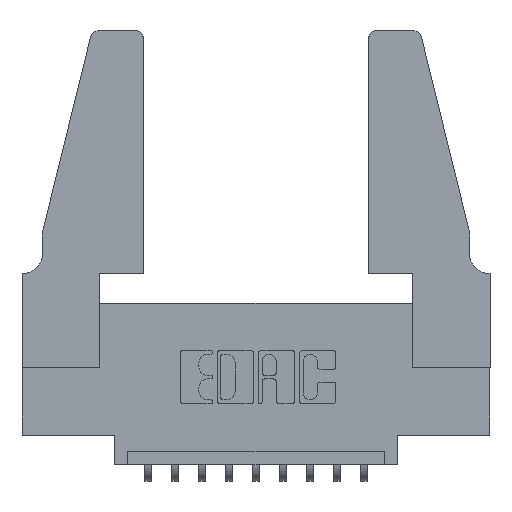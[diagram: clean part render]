
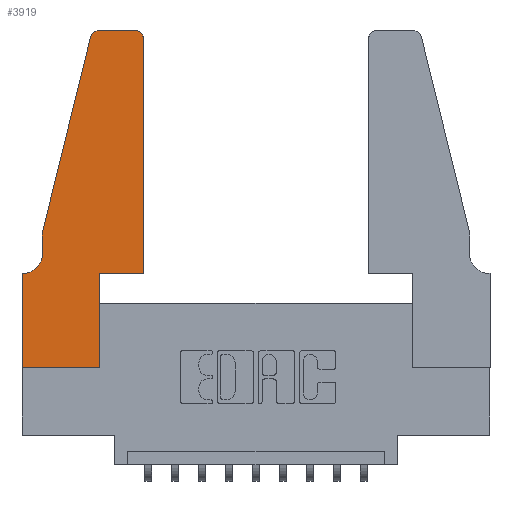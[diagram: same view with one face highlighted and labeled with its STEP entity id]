
A CAD part, top view. The second image highlights one B-rep face of the part: STEP entity #3919.
In plain terms, the highlighted planar face has unit normal (0, 0, 1).
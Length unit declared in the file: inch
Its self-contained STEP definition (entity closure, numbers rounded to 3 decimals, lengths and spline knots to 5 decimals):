
#287 = LINE ( 'NONE', #10560, #8342 ) ;
#307 = ORIENTED_EDGE ( 'NONE', *, *, #9730, .T. ) ;
#437 = VERTEX_POINT ( 'NONE', #11370 ) ;
#475 = VERTEX_POINT ( 'NONE', #1835 ) ;
#777 = LINE ( 'NONE', #6618, #8661 ) ;
#982 = LINE ( 'NONE', #2436, #11842 ) ;
#1007 = ORIENTED_EDGE ( 'NONE', *, *, #13517, .T. ) ;
#1078 = ORIENTED_EDGE ( 'NONE', *, *, #10433, .T. ) ;
#1210 = EDGE_CURVE ( 'NONE', #7350, #8159, #982, .T. ) ;
#1356 = CARTESIAN_POINT ( 'NONE',  ( 0.2865, 0.35, 0.37 ) ) ;
#1608 = CARTESIAN_POINT ( 'NONE',  ( 0., 0., 0.37 ) ) ;
#1835 = CARTESIAN_POINT ( 'NONE',  ( 0., 0.35, 0.37 ) ) ;
#1898 = FACE_OUTER_BOUND ( 'NONE', #8566, .T. ) ;
#2314 = DIRECTION ( 'NONE',  ( 0., 0., 1. ) ) ;
#2424 = DIRECTION ( 'NONE',  ( 0., -1., 0. ) ) ;
#2436 = CARTESIAN_POINT ( 'NONE',  ( 0.4505, 0.35, 0.37 ) ) ;
#2464 = EDGE_CURVE ( 'NONE', #13590, #475, #287, .T. ) ;
#2504 = VECTOR ( 'NONE', #5939, 39.37008 ) ;
#2513 = CARTESIAN_POINT ( 'NONE',  ( 0.0755, 0.5, 0.37 ) ) ;
#2754 = CARTESIAN_POINT ( 'NONE',  ( 0.284, 1.25, 0.37 ) ) ;
#2785 = ORIENTED_EDGE ( 'NONE', *, *, #2464, .T. ) ;
#3028 = DIRECTION ( 'NONE',  ( -1., 0., 0. ) ) ;
#3050 = AXIS2_PLACEMENT_3D ( 'NONE', #4557, #2314, #10827 ) ;
#3152 = CARTESIAN_POINT ( 'NONE',  ( 0.4505, 0.35, 0.37 ) ) ;
#3295 = CIRCLE ( 'NONE', #5211, 0.03 ) ;
#3298 = VERTEX_POINT ( 'NONE', #2754 ) ;
#3919 = ADVANCED_FACE ( 'NONE', ( #1898 ), #7598, .T. ) ;
#4323 = CARTESIAN_POINT ( 'NONE',  ( 0.4505, 1.22, 0.37 ) ) ;
#4397 = CARTESIAN_POINT ( 'NONE',  ( 0.284, 1.22, 0.37 ) ) ;
#4518 = VERTEX_POINT ( 'NONE', #5863 ) ;
#4557 = CARTESIAN_POINT ( 'NONE',  ( 0., 0.35, 0.37 ) ) ;
#4565 = DIRECTION ( 'NONE',  ( 0., 1., 0. ) ) ;
#4629 = DIRECTION ( 'NONE',  ( -0.239, -0.971, 0. ) ) ;
#4706 = EDGE_CURVE ( 'NONE', #11980, #3298, #4819, .T. ) ;
#4819 = LINE ( 'NONE', #10544, #2504 ) ;
#4822 = DIRECTION ( 'NONE',  ( 1., 0., 0. ) ) ;
#4834 = CARTESIAN_POINT ( 'NONE',  ( 0.4205, 1.25, 0.37 ) ) ;
#4905 = CARTESIAN_POINT ( 'NONE',  ( 0.0755, 0.5, 0.37 ) ) ;
#4990 = CARTESIAN_POINT ( 'NONE',  ( 0.25487, 1.22718, 0.37 ) ) ;
#5211 = AXIS2_PLACEMENT_3D ( 'NONE', #4397, #11756, #9801 ) ;
#5216 = DIRECTION ( 'NONE',  ( 0., 1., 0. ) ) ;
#5446 = VERTEX_POINT ( 'NONE', #8332 ) ;
#5470 = EDGE_CURVE ( 'NONE', #8159, #7039, #11714, .T. ) ;
#5863 = CARTESIAN_POINT ( 'NONE',  ( 0., 0., 0.37 ) ) ;
#5908 = AXIS2_PLACEMENT_3D ( 'NONE', #11105, #8009, #8155 ) ;
#5939 = DIRECTION ( 'NONE',  ( -1., 0., 0. ) ) ;
#6213 = LINE ( 'NONE', #4905, #8526 ) ;
#6260 = VERTEX_POINT ( 'NONE', #8687 ) ;
#6618 = CARTESIAN_POINT ( 'NONE',  ( 0., 0., 0.37 ) ) ;
#7039 = VERTEX_POINT ( 'NONE', #4323 ) ;
#7205 = ORIENTED_EDGE ( 'NONE', *, *, #4706, .T. ) ;
#7226 = LINE ( 'NONE', #1356, #11369 ) ;
#7256 = DIRECTION ( 'NONE',  ( 0., 0., 1. ) ) ;
#7350 = VERTEX_POINT ( 'NONE', #12616 ) ;
#7569 = VECTOR ( 'NONE', #4822, 39.37008 ) ;
#7598 = PLANE ( 'NONE',  #3050 ) ;
#7977 = EDGE_CURVE ( 'NONE', #11031, #5446, #13205, .T. ) ;
#8009 = DIRECTION ( 'NONE',  ( 0., 0., -1. ) ) ;
#8155 = DIRECTION ( 'NONE',  ( -1., 0., 0. ) ) ;
#8159 = VERTEX_POINT ( 'NONE', #12936 ) ;
#8284 = VECTOR ( 'NONE', #4629, 39.37008 ) ;
#8332 = CARTESIAN_POINT ( 'NONE',  ( 0.0755, 0.5, 0.37 ) ) ;
#8342 = VECTOR ( 'NONE', #3028, 39.37008 ) ;
#8404 = DIRECTION ( 'NONE',  ( 1., 0., 0. ) ) ;
#8526 = VECTOR ( 'NONE', #12279, 39.37008 ) ;
#8566 = EDGE_LOOP ( 'NONE', ( #7205, #9255, #9726, #11426, #9881, #2785, #1007, #11525, #1078, #8579, #12357, #307 ) ) ;
#8579 = ORIENTED_EDGE ( 'NONE', *, *, #1210, .T. ) ;
#8630 = AXIS2_PLACEMENT_3D ( 'NONE', #9353, #7256, #8404 ) ;
#8661 = VECTOR ( 'NONE', #2424, 39.37008 ) ;
#8687 = CARTESIAN_POINT ( 'NONE',  ( 0.0755, 0.42, 0.37 ) ) ;
#8921 = VECTOR ( 'NONE', #5216, 39.37008 ) ;
#9255 = ORIENTED_EDGE ( 'NONE', *, *, #10868, .T. ) ;
#9353 = CARTESIAN_POINT ( 'NONE',  ( 0.4205, 1.22, 0.37 ) ) ;
#9726 = ORIENTED_EDGE ( 'NONE', *, *, #7977, .T. ) ;
#9730 = EDGE_CURVE ( 'NONE', #7039, #11980, #9901, .T. ) ;
#9801 = DIRECTION ( 'NONE',  ( 1., 0., 0. ) ) ;
#9870 = EDGE_CURVE ( 'NONE', #4518, #437, #10537, .T. ) ;
#9881 = ORIENTED_EDGE ( 'NONE', *, *, #10649, .T. ) ;
#9901 = CIRCLE ( 'NONE', #8630, 0.03 ) ;
#10433 = EDGE_CURVE ( 'NONE', #437, #7350, #7226, .T. ) ;
#10537 = LINE ( 'NONE', #1608, #7569 ) ;
#10544 = CARTESIAN_POINT ( 'NONE',  ( 0.2605, 1.25, 0.37 ) ) ;
#10560 = CARTESIAN_POINT ( 'NONE',  ( 0.0755, 0.35, 0.37 ) ) ;
#10649 = EDGE_CURVE ( 'NONE', #6260, #13590, #11207, .T. ) ;
#10827 = DIRECTION ( 'NONE',  ( 1., 0., 0. ) ) ;
#10868 = EDGE_CURVE ( 'NONE', #3298, #11031, #3295, .T. ) ;
#11031 = VERTEX_POINT ( 'NONE', #4990 ) ;
#11105 = CARTESIAN_POINT ( 'NONE',  ( 0.0055, 0.42, 0.37 ) ) ;
#11207 = CIRCLE ( 'NONE', #5908, 0.07 ) ;
#11369 = VECTOR ( 'NONE', #4565, 39.37008 ) ;
#11370 = CARTESIAN_POINT ( 'NONE',  ( 0.2865, 0., 0.37 ) ) ;
#11426 = ORIENTED_EDGE ( 'NONE', *, *, #11704, .T. ) ;
#11525 = ORIENTED_EDGE ( 'NONE', *, *, #9870, .T. ) ;
#11704 = EDGE_CURVE ( 'NONE', #5446, #6260, #6213, .T. ) ;
#11714 = LINE ( 'NONE', #3152, #8921 ) ;
#11756 = DIRECTION ( 'NONE',  ( 0., 0., 1. ) ) ;
#11842 = VECTOR ( 'NONE', #12818, 39.37008 ) ;
#11867 = CARTESIAN_POINT ( 'NONE',  ( 0.0055, 0.35, 0.37 ) ) ;
#11980 = VERTEX_POINT ( 'NONE', #4834 ) ;
#12279 = DIRECTION ( 'NONE',  ( 0., -1., 0. ) ) ;
#12357 = ORIENTED_EDGE ( 'NONE', *, *, #5470, .T. ) ;
#12616 = CARTESIAN_POINT ( 'NONE',  ( 0.2865, 0.35, 0.37 ) ) ;
#12818 = DIRECTION ( 'NONE',  ( 1., 0., 0. ) ) ;
#12936 = CARTESIAN_POINT ( 'NONE',  ( 0.4505, 0.35, 0.37 ) ) ;
#13205 = LINE ( 'NONE', #2513, #8284 ) ;
#13517 = EDGE_CURVE ( 'NONE', #475, #4518, #777, .T. ) ;
#13590 = VERTEX_POINT ( 'NONE', #11867 ) ;
